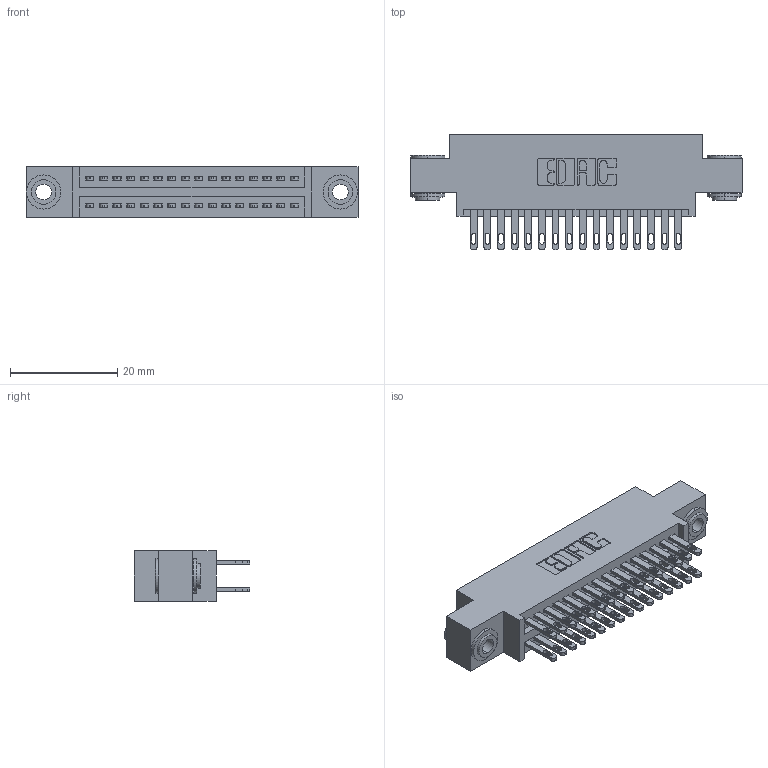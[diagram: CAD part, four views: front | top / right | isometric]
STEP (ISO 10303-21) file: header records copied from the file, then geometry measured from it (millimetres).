
FILE_DESCRIPTION (( 'STEP AP203' ), '1' );
FILE_NAME ('895-032-500-803.STEP', '2020-09-25T19:40:24', ( '' ), ( '' ), 'SwSTEP 2.0', 'SolidWorks 2020', '' );
FILE_SCHEMA (( 'CONFIG_CONTROL_DESIGN' ));
Length unit declared in the file: inch
Products named in the file (4): 345-292-001_345-293-100; 895-032-500-803; 845 Part_0.170 Offset - 0.156 Dia-TH; 345-250-002_345-250-002-102
Assembly tree (35 placements, depth 2):
  895-032-500-803
    845 Part_0.170 Offset - 0.156 Dia-TH
    345-292-001_345-293-100  x32
    345-250-002_345-250-002-102  x2
Bounding box: 61.85 x 21.51 x 9.4 mm (x, y, z)
Volume: 5770.5 mm3; surface area: 8701 mm2
Topology: 35 solids, 35 shells, 1640 faces, 4941 edges, 3290 vertices
Faces by surface type: plane 958, cylinder 674, cone 8
Entity records: 16766 total; most frequent: CARTESIAN_POINT 2811, ORIENTED_EDGE 2738, DIRECTION 2543, EDGE_CURVE 1369, LINE 1145, VECTOR 1145, VERTEX_POINT 910, AXIS2_PLACEMENT_3D 699
